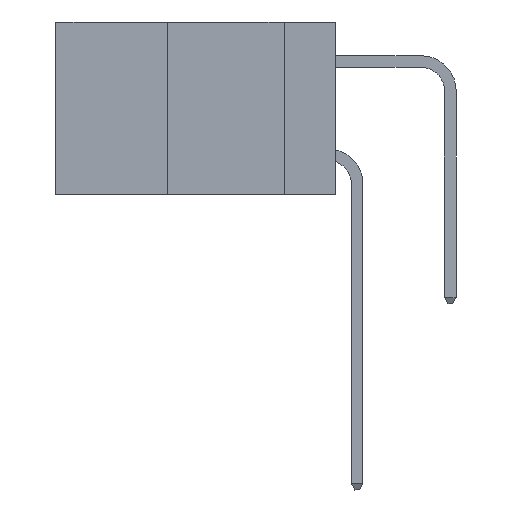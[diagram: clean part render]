
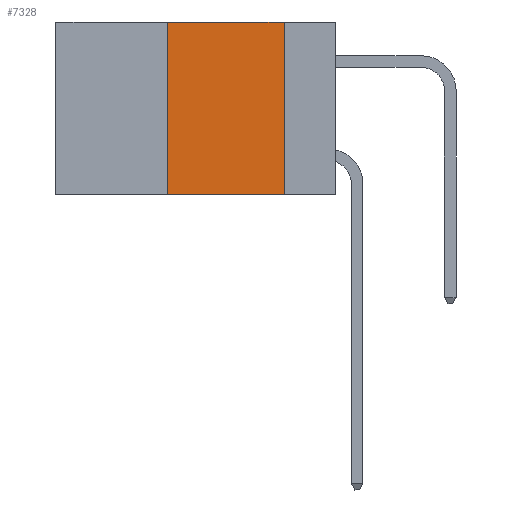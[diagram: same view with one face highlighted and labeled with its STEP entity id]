
A CAD part, left-side view. The second image highlights one B-rep face of the part: STEP entity #7328.
In plain terms, the highlighted planar face has unit normal (-1, 0, 0).
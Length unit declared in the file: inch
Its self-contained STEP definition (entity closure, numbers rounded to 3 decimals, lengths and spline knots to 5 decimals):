
#1828 = EDGE_CURVE ( 'NONE', #16947, #13757, #2130, .T. ) ;
#2130 = LINE ( 'NONE', #36390, #29528 ) ;
#3658 = ORIENTED_EDGE ( 'NONE', *, *, #15551, .F. ) ;
#5342 = LINE ( 'NONE', #27984, #20722 ) ;
#5644 = LINE ( 'NONE', #21886, #28224 ) ;
#6994 = PLANE ( 'NONE',  #22543 ) ;
#7328 = ADVANCED_FACE ( 'NONE', ( #18319 ), #6994, .F. ) ;
#9011 = EDGE_CURVE ( 'NONE', #30739, #21258, #5644, .T. ) ;
#9785 = CARTESIAN_POINT ( 'NONE',  ( 0., 0.36, -0.37 ) ) ;
#9825 = EDGE_LOOP ( 'NONE', ( #32735, #3658, #35628, #11166 ) ) ;
#9945 = DIRECTION ( 'NONE',  ( 0., 0., -1. ) ) ;
#11166 = ORIENTED_EDGE ( 'NONE', *, *, #25806, .T. ) ;
#13757 = VERTEX_POINT ( 'NONE', #15501 ) ;
#15501 = CARTESIAN_POINT ( 'NONE',  ( 0., 0.11, -0.37 ) ) ;
#15551 = EDGE_CURVE ( 'NONE', #21258, #16947, #5342, .T. ) ;
#16947 = VERTEX_POINT ( 'NONE', #34826 ) ;
#18319 = FACE_OUTER_BOUND ( 'NONE', #9825, .T. ) ;
#19099 = DIRECTION ( 'NONE',  ( 1., 0., 0. ) ) ;
#20716 = CARTESIAN_POINT ( 'NONE',  ( 0., 0.36, 0. ) ) ;
#20722 = VECTOR ( 'NONE', #21925, 39.37008 ) ;
#21258 = VERTEX_POINT ( 'NONE', #20716 ) ;
#21886 = CARTESIAN_POINT ( 'NONE',  ( 0., 0.36, 0. ) ) ;
#21925 = DIRECTION ( 'NONE',  ( 0., -1., 0. ) ) ;
#22543 = AXIS2_PLACEMENT_3D ( 'NONE', #34824, #19099, #9945 ) ;
#25806 = EDGE_CURVE ( 'NONE', #30739, #13757, #26135, .T. ) ;
#26135 = LINE ( 'NONE', #31580, #33860 ) ;
#27984 = CARTESIAN_POINT ( 'NONE',  ( 0., 0.6, 0. ) ) ;
#28061 = DIRECTION ( 'NONE',  ( 0., 0., 1. ) ) ;
#28224 = VECTOR ( 'NONE', #28061, 39.37008 ) ;
#29528 = VECTOR ( 'NONE', #37056, 39.37008 ) ;
#30739 = VERTEX_POINT ( 'NONE', #9785 ) ;
#31580 = CARTESIAN_POINT ( 'NONE',  ( 0., 0.6, -0.37 ) ) ;
#32735 = ORIENTED_EDGE ( 'NONE', *, *, #1828, .F. ) ;
#33860 = VECTOR ( 'NONE', #34541, 39.37008 ) ;
#34541 = DIRECTION ( 'NONE',  ( 0., -1., 0. ) ) ;
#34824 = CARTESIAN_POINT ( 'NONE',  ( 0., 0.6, 0. ) ) ;
#34826 = CARTESIAN_POINT ( 'NONE',  ( 0., 0.11, 0. ) ) ;
#35628 = ORIENTED_EDGE ( 'NONE', *, *, #9011, .F. ) ;
#36390 = CARTESIAN_POINT ( 'NONE',  ( 0., 0.11, 0. ) ) ;
#37056 = DIRECTION ( 'NONE',  ( 0., 0., -1. ) ) ;
